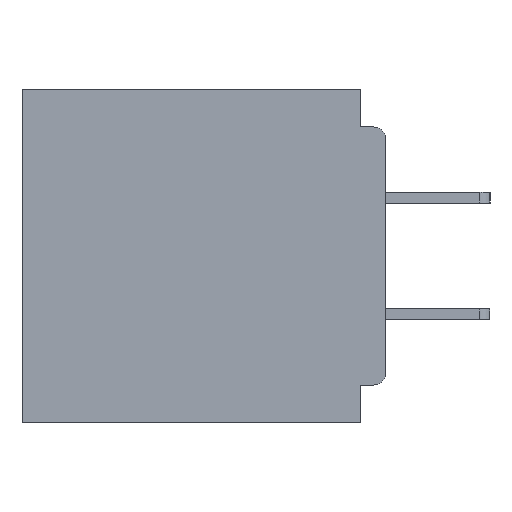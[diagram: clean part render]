
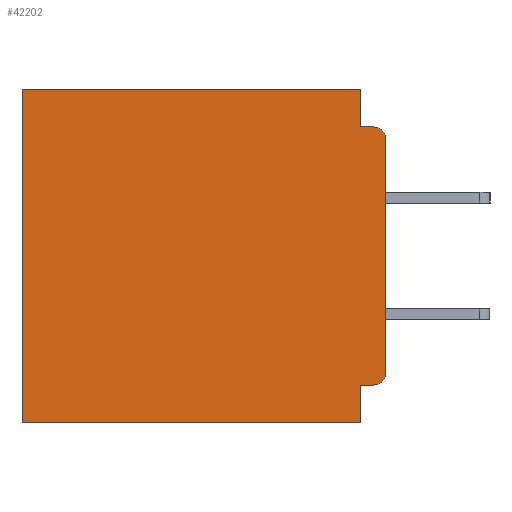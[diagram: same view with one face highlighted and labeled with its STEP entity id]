
A CAD part, left-side view. The second image highlights one B-rep face of the part: STEP entity #42202.
In plain terms, the highlighted planar face has unit normal (-1, 0, 0).
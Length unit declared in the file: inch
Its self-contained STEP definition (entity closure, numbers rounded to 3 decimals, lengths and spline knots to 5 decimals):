
#23 = EDGE_CURVE ( 'NONE', #20982, #1606, #17301, .T. ) ;
#271 = DIRECTION ( 'NONE',  ( 0., -1., 0. ) ) ;
#1086 = DIRECTION ( 'NONE',  ( 1., 0., 0. ) ) ;
#1606 = VERTEX_POINT ( 'NONE', #38368 ) ;
#2237 = VERTEX_POINT ( 'NONE', #56582 ) ;
#2586 = CARTESIAN_POINT ( 'NONE',  ( 0.3, 0.031, -0.045 ) ) ;
#2713 = EDGE_CURVE ( 'NONE', #13245, #1606, #11334, .T. ) ;
#3739 = EDGE_CURVE ( 'NONE', #20182, #16027, #54626, .T. ) ;
#4020 = DIRECTION ( 'NONE',  ( 0., 0., -1. ) ) ;
#5369 = VECTOR ( 'NONE', #4020, 39.37008 ) ;
#5424 = ORIENTED_EDGE ( 'NONE', *, *, #31838, .F. ) ;
#8245 = ORIENTED_EDGE ( 'NONE', *, *, #49042, .T. ) ;
#9724 = DIRECTION ( 'NONE',  ( 0., 0., -1. ) ) ;
#9731 = DIRECTION ( 'NONE',  ( -1., 0., 0. ) ) ;
#9851 = VERTEX_POINT ( 'NONE', #26882 ) ;
#11097 = VECTOR ( 'NONE', #36231, 39.37008 ) ;
#11263 = CARTESIAN_POINT ( 'NONE',  ( 0.3, 0.031, -0.355 ) ) ;
#11334 = LINE ( 'NONE', #24342, #35123 ) ;
#12861 = ORIENTED_EDGE ( 'NONE', *, *, #36879, .F. ) ;
#13058 = CARTESIAN_POINT ( 'NONE',  ( 0.3, 0.031, 0. ) ) ;
#13245 = VERTEX_POINT ( 'NONE', #42987 ) ;
#13553 = EDGE_CURVE ( 'NONE', #15446, #16027, #39856, .T. ) ;
#14232 = CARTESIAN_POINT ( 'NONE',  ( 0.3, 0., -0.4 ) ) ;
#15446 = VERTEX_POINT ( 'NONE', #2586 ) ;
#15902 = VECTOR ( 'NONE', #22140, 39.37008 ) ;
#16027 = VERTEX_POINT ( 'NONE', #24668 ) ;
#17301 = LINE ( 'NONE', #51986, #15902 ) ;
#18461 = ORIENTED_EDGE ( 'NONE', *, *, #55116, .F. ) ;
#19017 = CARTESIAN_POINT ( 'NONE',  ( 0.3, 0.015, -0.06 ) ) ;
#19752 = EDGE_LOOP ( 'NONE', ( #5424, #45356, #55722, #18461, #8245, #26014, #53700, #22653, #12861, #35222 ) ) ;
#20182 = VERTEX_POINT ( 'NONE', #26280 ) ;
#20982 = VERTEX_POINT ( 'NONE', #23978 ) ;
#21404 = EDGE_CURVE ( 'NONE', #27893, #20982, #43528, .T. ) ;
#22140 = DIRECTION ( 'NONE',  ( 0., 1., 0. ) ) ;
#22653 = ORIENTED_EDGE ( 'NONE', *, *, #21404, .F. ) ;
#22983 = LINE ( 'NONE', #31775, #11097 ) ;
#23448 = PLANE ( 'NONE',  #53828 ) ;
#23978 = CARTESIAN_POINT ( 'NONE',  ( 0.3, 0.031, -0.4 ) ) ;
#24227 = AXIS2_PLACEMENT_3D ( 'NONE', #19017, #41213, #50568 ) ;
#24342 = CARTESIAN_POINT ( 'NONE',  ( 0.3, 0.437, -0.4 ) ) ;
#24668 = CARTESIAN_POINT ( 'NONE',  ( 0.3, 0.015, -0.045 ) ) ;
#25342 = AXIS2_PLACEMENT_3D ( 'NONE', #36472, #9731, #40996 ) ;
#26014 = ORIENTED_EDGE ( 'NONE', *, *, #2713, .T. ) ;
#26280 = CARTESIAN_POINT ( 'NONE',  ( 0.3, 0., -0.06 ) ) ;
#26882 = CARTESIAN_POINT ( 'NONE',  ( 0.3, 0.031, 0. ) ) ;
#27893 = VERTEX_POINT ( 'NONE', #11263 ) ;
#28808 = CARTESIAN_POINT ( 'NONE',  ( 0.3, 0., -0.34 ) ) ;
#31775 = CARTESIAN_POINT ( 'NONE',  ( 0.3, 0., -0.355 ) ) ;
#31838 = EDGE_CURVE ( 'NONE', #20182, #55474, #51365, .T. ) ;
#32429 = DIRECTION ( 'NONE',  ( 0., 0., -1. ) ) ;
#33581 = EDGE_CURVE ( 'NONE', #2237, #55474, #42017, .T. ) ;
#35123 = VECTOR ( 'NONE', #58029, 39.37008 ) ;
#35222 = ORIENTED_EDGE ( 'NONE', *, *, #33581, .T. ) ;
#35857 = DIRECTION ( 'NONE',  ( 0., 0., -1. ) ) ;
#36231 = DIRECTION ( 'NONE',  ( 0., 1., 0. ) ) ;
#36472 = CARTESIAN_POINT ( 'NONE',  ( 0.3, 0.015, -0.34 ) ) ;
#36879 = EDGE_CURVE ( 'NONE', #2237, #27893, #22983, .T. ) ;
#37009 = VECTOR ( 'NONE', #271, 39.37008 ) ;
#38368 = CARTESIAN_POINT ( 'NONE',  ( 0.3, 0.437, -0.4 ) ) ;
#39436 = VECTOR ( 'NONE', #9724, 39.37008 ) ;
#39856 = LINE ( 'NONE', #40579, #37009 ) ;
#40348 = VECTOR ( 'NONE', #50626, 39.37008 ) ;
#40579 = CARTESIAN_POINT ( 'NONE',  ( 0.3, 0., -0.045 ) ) ;
#40996 = DIRECTION ( 'NONE',  ( 0., 0., -1. ) ) ;
#41213 = DIRECTION ( 'NONE',  ( -1., 0., 0. ) ) ;
#42017 = CIRCLE ( 'NONE', #25342, 0.015 ) ;
#42098 = VECTOR ( 'NONE', #35857, 39.37008 ) ;
#42202 = ADVANCED_FACE ( 'NONE', ( #53981 ), #23448, .F. ) ;
#42987 = CARTESIAN_POINT ( 'NONE',  ( 0.3, 0.437, 0. ) ) ;
#43528 = LINE ( 'NONE', #49218, #42098 ) ;
#45356 = ORIENTED_EDGE ( 'NONE', *, *, #3739, .T. ) ;
#46128 = CARTESIAN_POINT ( 'NONE',  ( 0.3, 0., 0. ) ) ;
#49042 = EDGE_CURVE ( 'NONE', #9851, #13245, #52323, .T. ) ;
#49218 = CARTESIAN_POINT ( 'NONE',  ( 0.3, 0.031, -0.4 ) ) ;
#50568 = DIRECTION ( 'NONE',  ( 0., 0., -1. ) ) ;
#50626 = DIRECTION ( 'NONE',  ( 0., 1., 0. ) ) ;
#51365 = LINE ( 'NONE', #14232, #39436 ) ;
#51615 = LINE ( 'NONE', #13058, #5369 ) ;
#51986 = CARTESIAN_POINT ( 'NONE',  ( 0.3, 0., -0.4 ) ) ;
#52323 = LINE ( 'NONE', #46128, #40348 ) ;
#53700 = ORIENTED_EDGE ( 'NONE', *, *, #23, .F. ) ;
#53828 = AXIS2_PLACEMENT_3D ( 'NONE', #54770, #1086, #32429 ) ;
#53981 = FACE_OUTER_BOUND ( 'NONE', #19752, .T. ) ;
#54626 = CIRCLE ( 'NONE', #24227, 0.015 ) ;
#54770 = CARTESIAN_POINT ( 'NONE',  ( 0.3, 0., -0.4 ) ) ;
#55116 = EDGE_CURVE ( 'NONE', #9851, #15446, #51615, .T. ) ;
#55474 = VERTEX_POINT ( 'NONE', #28808 ) ;
#55722 = ORIENTED_EDGE ( 'NONE', *, *, #13553, .F. ) ;
#56582 = CARTESIAN_POINT ( 'NONE',  ( 0.3, 0.015, -0.355 ) ) ;
#58029 = DIRECTION ( 'NONE',  ( 0., 0., -1. ) ) ;
